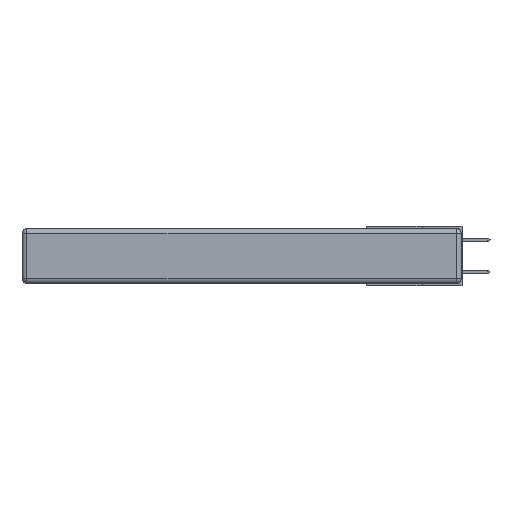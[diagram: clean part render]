
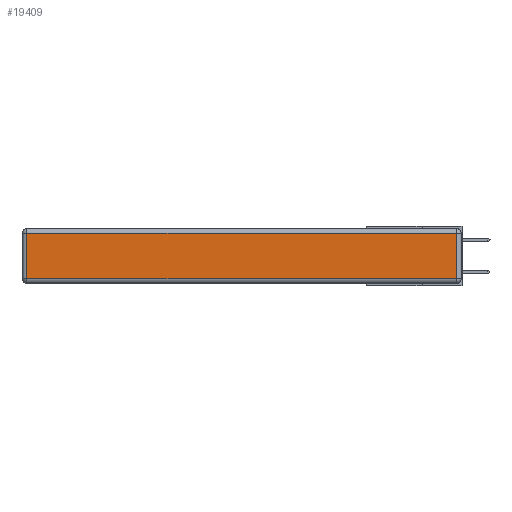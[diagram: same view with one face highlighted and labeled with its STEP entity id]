
A CAD part, left-side view. The second image highlights one B-rep face of the part: STEP entity #19409.
In plain terms, the highlighted planar face has unit normal (-1, 0, 0).
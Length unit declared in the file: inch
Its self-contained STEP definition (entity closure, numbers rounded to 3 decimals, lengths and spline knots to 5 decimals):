
#541 = DIRECTION ( 'NONE',  ( 0., 0., 1. ) ) ;
#1144 = VERTEX_POINT ( 'NONE', #12276 ) ;
#1180 = EDGE_LOOP ( 'NONE', ( #1418, #20892, #24591, #19397 ) ) ;
#1418 = ORIENTED_EDGE ( 'NONE', *, *, #13104, .T. ) ;
#1789 = VECTOR ( 'NONE', #24544, 39.37008 ) ;
#2444 = DIRECTION ( 'NONE',  ( 0., 1., 0. ) ) ;
#3695 = VECTOR ( 'NONE', #12481, 39.37008 ) ;
#3866 = EDGE_CURVE ( 'NONE', #23518, #1144, #10289, .T. ) ;
#5054 = CARTESIAN_POINT ( 'NONE',  ( 0., 2.72, -0.313 ) ) ;
#5358 = EDGE_CURVE ( 'NONE', #1144, #24080, #18441, .T. ) ;
#7804 = CARTESIAN_POINT ( 'NONE',  ( 0., 2.72, -0.343 ) ) ;
#7828 = VECTOR ( 'NONE', #2444, 39.37008 ) ;
#8838 = LINE ( 'NONE', #24098, #3695 ) ;
#9673 = DIRECTION ( 'NONE',  ( 0., 0., -1. ) ) ;
#10289 = LINE ( 'NONE', #20733, #1789 ) ;
#12276 = CARTESIAN_POINT ( 'NONE',  ( 0., 0.03, -0.03 ) ) ;
#12481 = DIRECTION ( 'NONE',  ( 0., -1., 0. ) ) ;
#12741 = CARTESIAN_POINT ( 'NONE',  ( 0., 0.03, -0.313 ) ) ;
#12923 = FACE_OUTER_BOUND ( 'NONE', #1180, .T. ) ;
#13104 = EDGE_CURVE ( 'NONE', #15084, #23518, #8838, .T. ) ;
#14020 = CARTESIAN_POINT ( 'NONE',  ( 0., 0., -0.343 ) ) ;
#15084 = VERTEX_POINT ( 'NONE', #5054 ) ;
#15326 = LINE ( 'NONE', #7804, #19826 ) ;
#15703 = AXIS2_PLACEMENT_3D ( 'NONE', #14020, #19596, #541 ) ;
#15887 = PLANE ( 'NONE',  #15703 ) ;
#16426 = CARTESIAN_POINT ( 'NONE',  ( 0., 2.75, -0.03 ) ) ;
#18441 = LINE ( 'NONE', #16426, #7828 ) ;
#19397 = ORIENTED_EDGE ( 'NONE', *, *, #21643, .T. ) ;
#19409 = ADVANCED_FACE ( 'NONE', ( #12923 ), #15887, .T. ) ;
#19596 = DIRECTION ( 'NONE',  ( -1., 0., 0. ) ) ;
#19826 = VECTOR ( 'NONE', #9673, 39.37008 ) ;
#20733 = CARTESIAN_POINT ( 'NONE',  ( 0., 0.03, -0.343 ) ) ;
#20892 = ORIENTED_EDGE ( 'NONE', *, *, #3866, .T. ) ;
#21643 = EDGE_CURVE ( 'NONE', #24080, #15084, #15326, .T. ) ;
#23502 = CARTESIAN_POINT ( 'NONE',  ( 0., 2.72, -0.03 ) ) ;
#23518 = VERTEX_POINT ( 'NONE', #12741 ) ;
#24080 = VERTEX_POINT ( 'NONE', #23502 ) ;
#24098 = CARTESIAN_POINT ( 'NONE',  ( 0., 0., -0.313 ) ) ;
#24544 = DIRECTION ( 'NONE',  ( 0., 0., 1. ) ) ;
#24591 = ORIENTED_EDGE ( 'NONE', *, *, #5358, .T. ) ;
